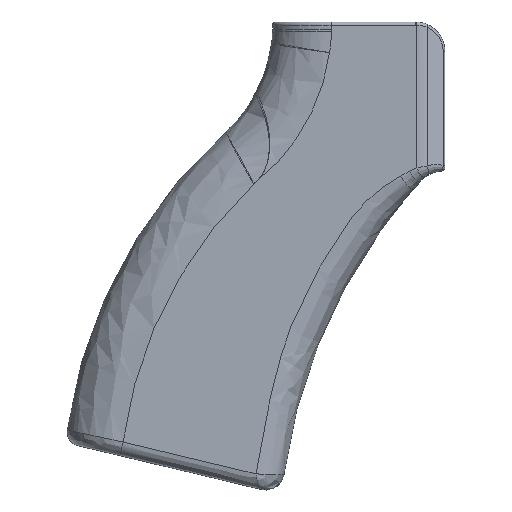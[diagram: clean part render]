
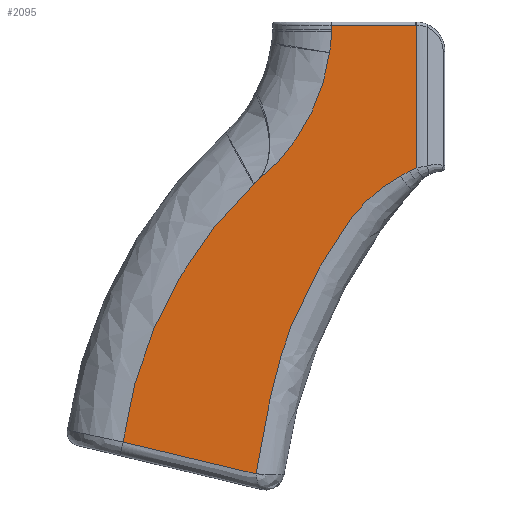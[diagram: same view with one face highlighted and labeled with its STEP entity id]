
A CAD part, left-side view. The second image highlights one B-rep face of the part: STEP entity #2095.
In plain terms, the highlighted planar face has unit normal (-1, 0, 0).
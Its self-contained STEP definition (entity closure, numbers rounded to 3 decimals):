
#173=B_SPLINE_CURVE_WITH_KNOTS('',3,(#5453,#5454,#5455,#5456),
 .UNSPECIFIED.,.F.,.F.,(4,4),(0.191,3.141),
 .UNSPECIFIED.);
#174=B_SPLINE_CURVE_WITH_KNOTS('',3,(#5458,#5459,#5460,#5461,#5462,#5463,
#5464,#5465,#5466,#5467,#5468,#5469,#5470,#5471),.UNSPECIFIED.,.F.,.F.,
(4,1,1,1,1,1,1,1,1,1,1,4),(1.002,1.53,2.059,
2.587,3.115,4.172,4.701,5.229,
6.286,7.343,7.871,8.399),
 .UNSPECIFIED.);
#175=B_SPLINE_CURVE_WITH_KNOTS('',3,(#5473,#5474,#5475,#5476,#5477,#5478,
#5479,#5480,#5481,#5482,#5483,#5484,#5485,#5486,#5487,#5488,#5489,#5490,
#5491,#5492,#5493,#5494,#5495,#5496,#5497,#5498),.UNSPECIFIED.,.F.,.F.,
(4,1,1,1,1,1,1,1,1,1,1,1,1,1,1,1,1,1,1,1,1,1,1,4),(0.775,0.789,
0.801,0.812,0.823,0.834,
0.845,0.856,0.867,0.878,0.888,
0.899,0.92,0.933,0.94,
0.947,0.954,0.961,0.968,
0.974,0.981,0.988,0.995,
1.002),.UNSPECIFIED.);
#176=B_SPLINE_CURVE_WITH_KNOTS('',3,(#5499,#5500,#5501,#5502,#5503,#5504,
#5505,#5506,#5507),.UNSPECIFIED.,.F.,.F.,(4,1,1,1,1,1,4),(0.589,
0.592,0.608,0.625,0.725,
0.769,0.775),.UNSPECIFIED.);
#256=PLANE('',#2297);
#371=FACE_OUTER_BOUND('',#516,.T.);
#516=EDGE_LOOP('',(#1821,#1822,#1823,#1824,#1825,#1826,#1827,#1828,#1829,
#1830,#1831,#1832));
#609=CIRCLE('',#2270,43.201);
#615=CIRCLE('',#2283,26.692);
#620=CIRCLE('',#2298,93.986);
#621=CIRCLE('',#2299,5.65);
#725=LINE('',#5021,#846);
#735=LINE('',#5430,#856);
#738=LINE('',#5449,#859);
#739=LINE('',#5450,#860);
#846=VECTOR('',#2703,10.);
#856=VECTOR('',#2739,10.);
#859=VECTOR('',#2748,10.);
#860=VECTOR('',#2749,10.);
#994=VERTEX_POINT('',#4874);
#1000=VERTEX_POINT('',#4943);
#1002=VERTEX_POINT('',#4955);
#1015=VERTEX_POINT('',#5019);
#1016=VERTEX_POINT('',#5020);
#1028=VERTEX_POINT('',#5423);
#1030=VERTEX_POINT('',#5429);
#1034=VERTEX_POINT('',#5447);
#1035=VERTEX_POINT('',#5448);
#1036=VERTEX_POINT('',#5452);
#1037=VERTEX_POINT('',#5457);
#1038=VERTEX_POINT('',#5472);
#1259=EDGE_CURVE('',#1002,#1000,#609,.T.);
#1278=EDGE_CURVE('',#1015,#1016,#725,.T.);
#1283=EDGE_CURVE('',#1015,#1002,#615,.T.);
#1305=EDGE_CURVE('',#1028,#1030,#735,.T.);
#1311=EDGE_CURVE('',#1034,#1035,#738,.T.);
#1312=EDGE_CURVE('',#1016,#1034,#739,.T.);
#1313=EDGE_CURVE('',#1000,#994,#620,.T.);
#1314=EDGE_CURVE('',#1036,#994,#173,.T.);
#1315=EDGE_CURVE('',#1037,#1036,#174,.T.);
#1316=EDGE_CURVE('',#1038,#1037,#175,.T.);
#1317=EDGE_CURVE('',#1030,#1038,#176,.T.);
#1318=EDGE_CURVE('',#1035,#1028,#621,.T.);
#1821=ORIENTED_EDGE('',*,*,#1311,.F.);
#1822=ORIENTED_EDGE('',*,*,#1312,.F.);
#1823=ORIENTED_EDGE('',*,*,#1278,.F.);
#1824=ORIENTED_EDGE('',*,*,#1283,.T.);
#1825=ORIENTED_EDGE('',*,*,#1259,.T.);
#1826=ORIENTED_EDGE('',*,*,#1313,.T.);
#1827=ORIENTED_EDGE('',*,*,#1314,.F.);
#1828=ORIENTED_EDGE('',*,*,#1315,.F.);
#1829=ORIENTED_EDGE('',*,*,#1316,.F.);
#1830=ORIENTED_EDGE('',*,*,#1317,.F.);
#1831=ORIENTED_EDGE('',*,*,#1305,.F.);
#1832=ORIENTED_EDGE('',*,*,#1318,.F.);
#2095=ADVANCED_FACE('',(#371),#256,.T.);
#2270=AXIS2_PLACEMENT_3D('',#4956,#2668,#2669);
#2283=AXIS2_PLACEMENT_3D('',#5092,#2707,#2708);
#2297=AXIS2_PLACEMENT_3D('',#5446,#2746,#2747);
#2298=AXIS2_PLACEMENT_3D('',#5451,#2750,#2751);
#2299=AXIS2_PLACEMENT_3D('',#5508,#2752,#2753);
#2668=DIRECTION('center_axis',(1.,0.,0.));
#2669=DIRECTION('ref_axis',(0.,-1.,0.018));
#2703=DIRECTION('',(0.,0.,1.));
#2707=DIRECTION('center_axis',(1.,0.,0.));
#2708=DIRECTION('ref_axis',(0.,-1.,0.));
#2739=DIRECTION('',(0.,0.,-1.));
#2746=DIRECTION('center_axis',(-1.,0.,0.));
#2747=DIRECTION('ref_axis',(0.,-1.,0.));
#2748=DIRECTION('',(0.,-1.,0.));
#2749=DIRECTION('',(0.,0.,1.));
#2750=DIRECTION('center_axis',(-1.,0.,0.));
#2751=DIRECTION('ref_axis',(0.,0.692,0.722));
#2752=DIRECTION('center_axis',(1.,0.,0.));
#2753=DIRECTION('ref_axis',(0.,-0.022,1.));
#4874=CARTESIAN_POINT('',(-11.49,-84.849,-99.847));
#4943=CARTESIAN_POINT('',(-11.49,-113.026,-44.17));
#4955=CARTESIAN_POINT('',(-11.49,-129.39,-15.845));
#4956=CARTESIAN_POINT('Origin',(-11.49,-86.586,-10.005));
#5019=CARTESIAN_POINT('',(-11.49,-129.779,-11.303));
#5020=CARTESIAN_POINT('',(-11.49,-129.779,-10.793));
#5021=CARTESIAN_POINT('',(-11.49,-129.779,-9.218));
#5092=CARTESIAN_POINT('Origin',(-11.49,-103.088,-11.303));
#5423=CARTESIAN_POINT('',(-11.49,-148.206,-9.924));
#5429=CARTESIAN_POINT('',(-11.49,-148.206,-40.672));
#5430=CARTESIAN_POINT('',(-11.49,-148.206,-26.609));
#5446=CARTESIAN_POINT('Origin',(-11.49,27.424,-44.));
#5447=CARTESIAN_POINT('',(-11.49,-129.779,-9.918));
#5448=CARTESIAN_POINT('',(-11.49,-147.932,-9.918));
#5449=CARTESIAN_POINT('',(-11.49,-44.832,-9.918));
#5450=CARTESIAN_POINT('',(-11.49,-129.779,-9.218));
#5451=CARTESIAN_POINT('Origin',(-11.49,-178.041,-112.041));
#5452=CARTESIAN_POINT('',(-11.49,-113.539,-106.708));
#5453=CARTESIAN_POINT('Ctrl Pts',(-11.49,-113.539,-106.708));
#5454=CARTESIAN_POINT('Ctrl Pts',(-11.49,-103.975,-104.421));
#5455=CARTESIAN_POINT('Ctrl Pts',(-11.49,-94.419,-102.135));
#5456=CARTESIAN_POINT('Ctrl Pts',(-11.49,-84.849,-99.847));
#5457=CARTESIAN_POINT('',(-11.49,-144.719,-42.455));
#5458=CARTESIAN_POINT('Ctrl Pts',(-11.49,-144.719,-42.455));
#5459=CARTESIAN_POINT('Ctrl Pts',(-11.49,-143.256,-43.246));
#5460=CARTESIAN_POINT('Ctrl Pts',(-11.49,-140.389,-45.043));
#5461=CARTESIAN_POINT('Ctrl Pts',(-11.49,-136.477,-48.536));
#5462=CARTESIAN_POINT('Ctrl Pts',(-11.49,-133.146,-52.657));
#5463=CARTESIAN_POINT('Ctrl Pts',(-11.49,-129.218,-58.505));
#5464=CARTESIAN_POINT('Ctrl Pts',(-11.49,-125.76,-64.658));
#5465=CARTESIAN_POINT('Ctrl Pts',(-11.49,-122.666,-70.985));
#5466=CARTESIAN_POINT('Ctrl Pts',(-11.49,-119.921,-77.492));
#5467=CARTESIAN_POINT('Ctrl Pts',(-11.49,-117.555,-85.97));
#5468=CARTESIAN_POINT('Ctrl Pts',(-11.49,-115.681,-94.566));
#5469=CARTESIAN_POINT('Ctrl Pts',(-11.49,-114.284,-101.475));
#5470=CARTESIAN_POINT('Ctrl Pts',(-11.49,-113.766,-104.96));
#5471=CARTESIAN_POINT('Ctrl Pts',(-11.49,-113.539,-106.708));
#5472=CARTESIAN_POINT('',(-11.49,-146.608,-41.441));
#5473=CARTESIAN_POINT('Ctrl Pts',(-11.49,-146.608,-41.441));
#5474=CARTESIAN_POINT('Ctrl Pts',(-11.49,-146.568,-41.463));
#5475=CARTESIAN_POINT('Ctrl Pts',(-11.49,-146.496,-41.503));
#5476=CARTESIAN_POINT('Ctrl Pts',(-11.49,-146.393,-41.559));
#5477=CARTESIAN_POINT('Ctrl Pts',(-11.49,-146.3,-41.61));
#5478=CARTESIAN_POINT('Ctrl Pts',(-11.49,-146.207,-41.66));
#5479=CARTESIAN_POINT('Ctrl Pts',(-11.49,-146.115,-41.71));
#5480=CARTESIAN_POINT('Ctrl Pts',(-11.49,-146.024,-41.759));
#5481=CARTESIAN_POINT('Ctrl Pts',(-11.49,-145.933,-41.808));
#5482=CARTESIAN_POINT('Ctrl Pts',(-11.49,-145.843,-41.856));
#5483=CARTESIAN_POINT('Ctrl Pts',(-11.49,-145.753,-41.903));
#5484=CARTESIAN_POINT('Ctrl Pts',(-11.49,-145.665,-41.951));
#5485=CARTESIAN_POINT('Ctrl Pts',(-11.49,-145.549,-42.012));
#5486=CARTESIAN_POINT('Ctrl Pts',(-11.49,-145.424,-42.079));
#5487=CARTESIAN_POINT('Ctrl Pts',(-11.49,-145.309,-42.14));
#5488=CARTESIAN_POINT('Ctrl Pts',(-11.49,-145.233,-42.18));
#5489=CARTESIAN_POINT('Ctrl Pts',(-11.49,-145.175,-42.21));
#5490=CARTESIAN_POINT('Ctrl Pts',(-11.49,-145.118,-42.241));
#5491=CARTESIAN_POINT('Ctrl Pts',(-11.49,-145.061,-42.271));
#5492=CARTESIAN_POINT('Ctrl Pts',(-11.49,-145.004,-42.302));
#5493=CARTESIAN_POINT('Ctrl Pts',(-11.49,-144.947,-42.332));
#5494=CARTESIAN_POINT('Ctrl Pts',(-11.49,-144.89,-42.363));
#5495=CARTESIAN_POINT('Ctrl Pts',(-11.49,-144.833,-42.393));
#5496=CARTESIAN_POINT('Ctrl Pts',(-11.49,-144.776,-42.424));
#5497=CARTESIAN_POINT('Ctrl Pts',(-11.49,-144.738,-42.444));
#5498=CARTESIAN_POINT('Ctrl Pts',(-11.49,-144.719,-42.455));
#5499=CARTESIAN_POINT('Ctrl Pts',(-11.49,-148.206,-40.672));
#5500=CARTESIAN_POINT('Ctrl Pts',(-11.49,-148.197,-40.675));
#5501=CARTESIAN_POINT('Ctrl Pts',(-11.49,-148.139,-40.699));
#5502=CARTESIAN_POINT('Ctrl Pts',(-11.49,-148.034,-40.743));
#5503=CARTESIAN_POINT('Ctrl Pts',(-11.49,-147.643,-40.912));
#5504=CARTESIAN_POINT('Ctrl Pts',(-11.49,-147.18,-41.134));
#5505=CARTESIAN_POINT('Ctrl Pts',(-11.49,-146.761,-41.357));
#5506=CARTESIAN_POINT('Ctrl Pts',(-11.49,-146.623,-41.433));
#5507=CARTESIAN_POINT('Ctrl Pts',(-11.49,-146.608,-41.441));
#5508=CARTESIAN_POINT('Origin',(-11.49,-147.932,-15.568));
